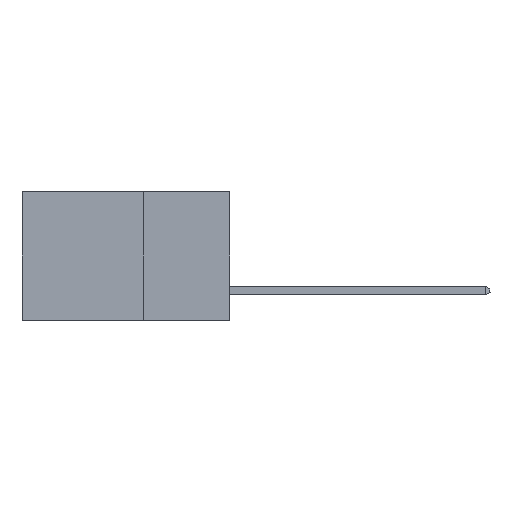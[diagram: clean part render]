
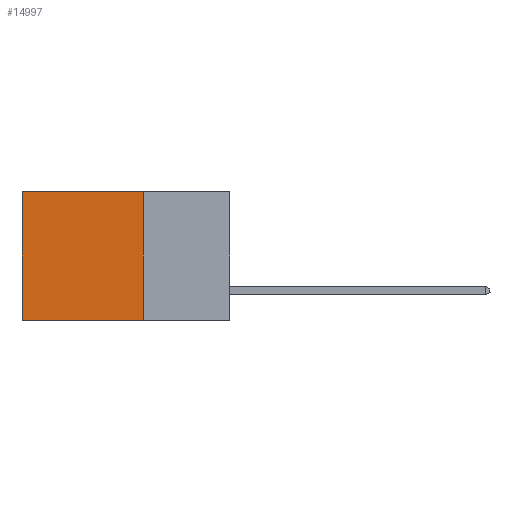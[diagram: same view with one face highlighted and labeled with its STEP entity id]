
A CAD part, left-side view. The second image highlights one B-rep face of the part: STEP entity #14997.
In plain terms, the highlighted planar face has unit normal (-1, 0, 0).
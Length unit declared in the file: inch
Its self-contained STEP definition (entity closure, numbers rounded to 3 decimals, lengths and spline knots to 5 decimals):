
#167 = CARTESIAN_POINT ( 'NONE',  ( 0.298, 0.25, -0.37 ) ) ;
#927 = DIRECTION ( 'NONE',  ( 1., 0., 0. ) ) ;
#1313 = VECTOR ( 'NONE', #6955, 39.37008 ) ;
#2144 = ORIENTED_EDGE ( 'NONE', *, *, #12786, .F. ) ;
#3816 = CARTESIAN_POINT ( 'NONE',  ( 0.298, 0.6, -0.37 ) ) ;
#4852 = CARTESIAN_POINT ( 'NONE',  ( 0.298, 0.25, -0.37 ) ) ;
#5098 = CARTESIAN_POINT ( 'NONE',  ( 0.298, 0.6, 0. ) ) ;
#6795 = EDGE_LOOP ( 'NONE', ( #23037, #2144, #14154, #16289 ) ) ;
#6937 = EDGE_CURVE ( 'NONE', #25998, #14434, #16422, .T. ) ;
#6955 = DIRECTION ( 'NONE',  ( 0., 1., 0. ) ) ;
#7986 = CARTESIAN_POINT ( 'NONE',  ( 0.298, 0.6, 0. ) ) ;
#7996 = VECTOR ( 'NONE', #29381, 39.37008 ) ;
#9502 = EDGE_CURVE ( 'NONE', #22706, #25998, #15221, .T. ) ;
#9648 = AXIS2_PLACEMENT_3D ( 'NONE', #12276, #927, #14888 ) ;
#11431 = LINE ( 'NONE', #167, #1313 ) ;
#12276 = CARTESIAN_POINT ( 'NONE',  ( 0.298, 0.25, 0. ) ) ;
#12786 = EDGE_CURVE ( 'NONE', #24756, #14434, #11431, .T. ) ;
#13050 = CARTESIAN_POINT ( 'NONE',  ( 0.298, 0.25, 0. ) ) ;
#14154 = ORIENTED_EDGE ( 'NONE', *, *, #15339, .F. ) ;
#14434 = VERTEX_POINT ( 'NONE', #3816 ) ;
#14888 = DIRECTION ( 'NONE',  ( 0., 0., -1. ) ) ;
#14984 = VECTOR ( 'NONE', #18918, 39.37008 ) ;
#14997 = ADVANCED_FACE ( 'NONE', ( #23956 ), #23910, .F. ) ;
#15221 = LINE ( 'NONE', #18840, #17381 ) ;
#15339 = EDGE_CURVE ( 'NONE', #22706, #24756, #23564, .T. ) ;
#16289 = ORIENTED_EDGE ( 'NONE', *, *, #9502, .T. ) ;
#16422 = LINE ( 'NONE', #7986, #14984 ) ;
#17381 = VECTOR ( 'NONE', #23495, 39.37008 ) ;
#18840 = CARTESIAN_POINT ( 'NONE',  ( 0.298, 0.25, 0. ) ) ;
#18918 = DIRECTION ( 'NONE',  ( 0., 0., -1. ) ) ;
#22706 = VERTEX_POINT ( 'NONE', #13050 ) ;
#23037 = ORIENTED_EDGE ( 'NONE', *, *, #6937, .T. ) ;
#23495 = DIRECTION ( 'NONE',  ( 0., 1., 0. ) ) ;
#23564 = LINE ( 'NONE', #29478, #7996 ) ;
#23910 = PLANE ( 'NONE',  #9648 ) ;
#23956 = FACE_OUTER_BOUND ( 'NONE', #6795, .T. ) ;
#24756 = VERTEX_POINT ( 'NONE', #4852 ) ;
#25998 = VERTEX_POINT ( 'NONE', #5098 ) ;
#29381 = DIRECTION ( 'NONE',  ( 0., 0., -1. ) ) ;
#29478 = CARTESIAN_POINT ( 'NONE',  ( 0.298, 0.25, 0. ) ) ;
